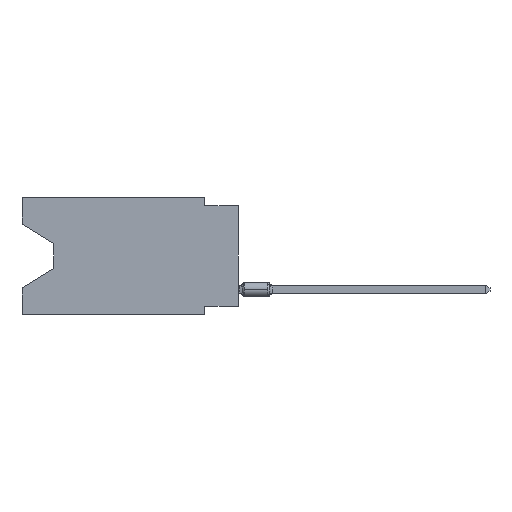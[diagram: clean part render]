
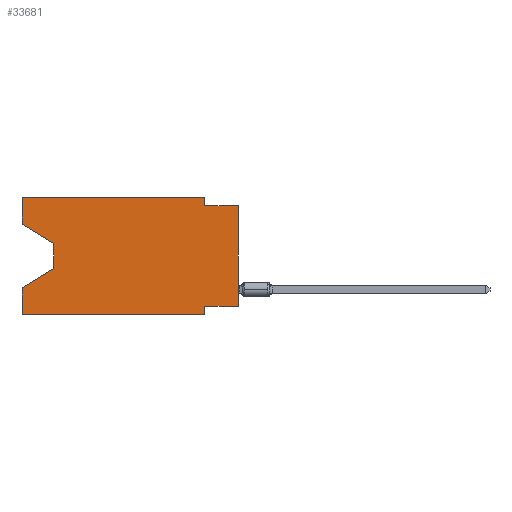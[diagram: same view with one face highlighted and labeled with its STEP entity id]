
A CAD part, left-side view. The second image highlights one B-rep face of the part: STEP entity #33681.
In plain terms, the highlighted planar face has unit normal (-1, 0, 0).
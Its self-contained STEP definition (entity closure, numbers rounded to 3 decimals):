
#533 = DIRECTION ( 'NONE',  ( 0., 0., -1. ) ) ;
#681 = VECTOR ( 'NONE', #13432, 1000. ) ;
#860 = EDGE_CURVE ( 'NONE', #36932, #20805, #29374, .T. ) ;
#1111 = CARTESIAN_POINT ( 'NONE',  ( 0., 16.383, -2.038 ) ) ;
#1652 = VERTEX_POINT ( 'NONE', #33388 ) ;
#2306 = FACE_OUTER_BOUND ( 'NONE', #18326, .T. ) ;
#2328 = ORIENTED_EDGE ( 'NONE', *, *, #20333, .F. ) ;
#2588 = LINE ( 'NONE', #9434, #16380 ) ;
#2741 = CARTESIAN_POINT ( 'NONE',  ( 0., 16.383, 0. ) ) ;
#2901 = CARTESIAN_POINT ( 'NONE',  ( 0., 0., -8.255 ) ) ;
#4205 = LINE ( 'NONE', #23647, #6800 ) ;
#5308 = LINE ( 'NONE', #35799, #35014 ) ;
#5671 = ORIENTED_EDGE ( 'NONE', *, *, #860, .T. ) ;
#5777 = DIRECTION ( 'NONE',  ( 0., -1., 0. ) ) ;
#6395 = CARTESIAN_POINT ( 'NONE',  ( 0., 16.383, -2.038 ) ) ;
#6619 = VERTEX_POINT ( 'NONE', #22943 ) ;
#6800 = VECTOR ( 'NONE', #7511, 1000. ) ;
#6918 = CARTESIAN_POINT ( 'NONE',  ( 0., 2.54, -8.89 ) ) ;
#7369 = LINE ( 'NONE', #33877, #13089 ) ;
#7511 = DIRECTION ( 'NONE',  ( 0., 0., 1. ) ) ;
#8273 = VECTOR ( 'NONE', #42508, 1000. ) ;
#8317 = DIRECTION ( 'NONE',  ( 0., 0., 1. ) ) ;
#8394 = ORIENTED_EDGE ( 'NONE', *, *, #39275, .F. ) ;
#9059 = ORIENTED_EDGE ( 'NONE', *, *, #26816, .F. ) ;
#9434 = CARTESIAN_POINT ( 'NONE',  ( 0., 2.54, -8.89 ) ) ;
#9474 = CARTESIAN_POINT ( 'NONE',  ( 0., 16.383, -8.89 ) ) ;
#9662 = CARTESIAN_POINT ( 'NONE',  ( 0., 0., -0.635 ) ) ;
#9909 = EDGE_CURVE ( 'NONE', #20805, #41952, #31102, .T. ) ;
#10018 = EDGE_CURVE ( 'NONE', #23732, #12599, #42509, .T. ) ;
#10536 = LINE ( 'NONE', #19799, #35438 ) ;
#10651 = CARTESIAN_POINT ( 'NONE',  ( 0., 13.97, -5.385 ) ) ;
#10974 = ORIENTED_EDGE ( 'NONE', *, *, #34784, .F. ) ;
#11997 = CARTESIAN_POINT ( 'NONE',  ( 0., 16.383, -8.89 ) ) ;
#12082 = CARTESIAN_POINT ( 'NONE',  ( 0., 16.383, 0. ) ) ;
#12400 = DIRECTION ( 'NONE',  ( 0., -1., 0. ) ) ;
#12477 = DIRECTION ( 'NONE',  ( 0., 0., -1. ) ) ;
#12599 = VERTEX_POINT ( 'NONE', #25648 ) ;
#12977 = LINE ( 'NONE', #9662, #681 ) ;
#13089 = VECTOR ( 'NONE', #533, 1000. ) ;
#13377 = CARTESIAN_POINT ( 'NONE',  ( 0., 13.97, -5.385 ) ) ;
#13432 = DIRECTION ( 'NONE',  ( 0., -1., 0. ) ) ;
#14246 = AXIS2_PLACEMENT_3D ( 'NONE', #2741, #15802, #12477 ) ;
#14589 = VECTOR ( 'NONE', #24892, 1000. ) ;
#14918 = EDGE_CURVE ( 'NONE', #6619, #1652, #5308, .T. ) ;
#15027 = ORIENTED_EDGE ( 'NONE', *, *, #14918, .F. ) ;
#15442 = DIRECTION ( 'NONE',  ( 0., 0., -1. ) ) ;
#15452 = VERTEX_POINT ( 'NONE', #6918 ) ;
#15802 = DIRECTION ( 'NONE',  ( 1., 0., 0. ) ) ;
#16054 = EDGE_CURVE ( 'NONE', #36794, #35510, #41861, .T. ) ;
#16156 = VECTOR ( 'NONE', #37574, 1000. ) ;
#16380 = VECTOR ( 'NONE', #15442, 1000. ) ;
#16476 = CARTESIAN_POINT ( 'NONE',  ( 0., 13.97, -3.505 ) ) ;
#17716 = LINE ( 'NONE', #10651, #16156 ) ;
#18326 = EDGE_LOOP ( 'NONE', ( #5671, #25411, #19317, #22827, #36266, #8394, #10974, #38179, #2328, #9059, #15027, #20700 ) ) ;
#19317 = ORIENTED_EDGE ( 'NONE', *, *, #30145, .T. ) ;
#19744 = VECTOR ( 'NONE', #22957, 1000. ) ;
#19799 = CARTESIAN_POINT ( 'NONE',  ( 0., 0., -8.255 ) ) ;
#20333 = EDGE_CURVE ( 'NONE', #39537, #35510, #12977, .T. ) ;
#20700 = ORIENTED_EDGE ( 'NONE', *, *, #27890, .F. ) ;
#20805 = VERTEX_POINT ( 'NONE', #16476 ) ;
#21577 = CARTESIAN_POINT ( 'NONE',  ( 0., 13.97, -3.505 ) ) ;
#22827 = ORIENTED_EDGE ( 'NONE', *, *, #10018, .F. ) ;
#22943 = CARTESIAN_POINT ( 'NONE',  ( 0., 16.383, 0. ) ) ;
#22957 = DIRECTION ( 'NONE',  ( 0., -0.855, -0.519 ) ) ;
#23647 = CARTESIAN_POINT ( 'NONE',  ( 0., 16.383, 0. ) ) ;
#23732 = VERTEX_POINT ( 'NONE', #9474 ) ;
#24566 = VECTOR ( 'NONE', #5777, 1000. ) ;
#24892 = DIRECTION ( 'NONE',  ( 0., 0., -1. ) ) ;
#25411 = ORIENTED_EDGE ( 'NONE', *, *, #9909, .T. ) ;
#25648 = CARTESIAN_POINT ( 'NONE',  ( 0., 16.383, -6.852 ) ) ;
#26816 = EDGE_CURVE ( 'NONE', #1652, #39537, #7369, .T. ) ;
#27890 = EDGE_CURVE ( 'NONE', #36932, #6619, #4205, .T. ) ;
#29046 = PLANE ( 'NONE',  #14246 ) ;
#29374 = LINE ( 'NONE', #6395, #19744 ) ;
#29384 = VERTEX_POINT ( 'NONE', #40378 ) ;
#29846 = EDGE_CURVE ( 'NONE', #23732, #15452, #39118, .T. ) ;
#30145 = EDGE_CURVE ( 'NONE', #41952, #12599, #17716, .T. ) ;
#31102 = LINE ( 'NONE', #21577, #14589 ) ;
#33388 = CARTESIAN_POINT ( 'NONE',  ( 0., 2.54, 0. ) ) ;
#33681 = ADVANCED_FACE ( 'NONE', ( #2306 ), #29046, .F. ) ;
#33877 = CARTESIAN_POINT ( 'NONE',  ( 0., 2.54, 0. ) ) ;
#34784 = EDGE_CURVE ( 'NONE', #36794, #29384, #10536, .T. ) ;
#35014 = VECTOR ( 'NONE', #12400, 1000. ) ;
#35438 = VECTOR ( 'NONE', #40521, 1000. ) ;
#35510 = VERTEX_POINT ( 'NONE', #39550 ) ;
#35799 = CARTESIAN_POINT ( 'NONE',  ( 0., 16.383, 0. ) ) ;
#36266 = ORIENTED_EDGE ( 'NONE', *, *, #29846, .T. ) ;
#36794 = VERTEX_POINT ( 'NONE', #2901 ) ;
#36932 = VERTEX_POINT ( 'NONE', #1111 ) ;
#37574 = DIRECTION ( 'NONE',  ( 0., 0.855, -0.519 ) ) ;
#37912 = CARTESIAN_POINT ( 'NONE',  ( 0., 2.54, -0.635 ) ) ;
#38179 = ORIENTED_EDGE ( 'NONE', *, *, #16054, .T. ) ;
#39118 = LINE ( 'NONE', #11997, #24566 ) ;
#39260 = VECTOR ( 'NONE', #8317, 1000. ) ;
#39275 = EDGE_CURVE ( 'NONE', #29384, #15452, #2588, .T. ) ;
#39431 = CARTESIAN_POINT ( 'NONE',  ( 0., 0., 0. ) ) ;
#39537 = VERTEX_POINT ( 'NONE', #37912 ) ;
#39550 = CARTESIAN_POINT ( 'NONE',  ( 0., 0., -0.635 ) ) ;
#40378 = CARTESIAN_POINT ( 'NONE',  ( 0., 2.54, -8.255 ) ) ;
#40521 = DIRECTION ( 'NONE',  ( 0., 1., 0. ) ) ;
#41861 = LINE ( 'NONE', #39431, #8273 ) ;
#41952 = VERTEX_POINT ( 'NONE', #13377 ) ;
#42508 = DIRECTION ( 'NONE',  ( 0., 0., 1. ) ) ;
#42509 = LINE ( 'NONE', #12082, #39260 ) ;
